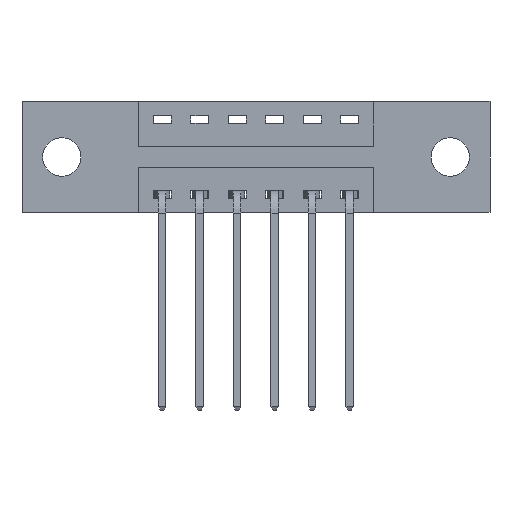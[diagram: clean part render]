
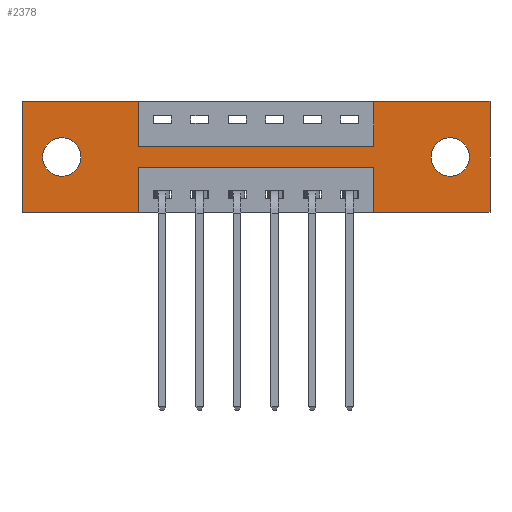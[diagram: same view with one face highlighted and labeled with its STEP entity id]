
A CAD part, front view. The second image highlights one B-rep face of the part: STEP entity #2378.
In plain terms, the highlighted planar face has unit normal (0, -1, 0).
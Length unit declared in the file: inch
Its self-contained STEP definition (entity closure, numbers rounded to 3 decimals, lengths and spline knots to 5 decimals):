
#19 = DIRECTION ( 'NONE',  ( 0., 0., -1. ) ) ;
#32 = CARTESIAN_POINT ( 'NONE',  ( 0., 0., -0.37 ) ) ;
#41 = VERTEX_POINT ( 'NONE', #8412 ) ;
#143 = CARTESIAN_POINT ( 'NONE',  ( 0.1325, 0., -0.249 ) ) ;
#238 = VERTEX_POINT ( 'NONE', #3917 ) ;
#343 = DIRECTION ( 'NONE',  ( 0., 1., 0. ) ) ;
#346 = VERTEX_POINT ( 'NONE', #7592 ) ;
#360 = ORIENTED_EDGE ( 'NONE', *, *, #2982, .F. ) ;
#462 = VERTEX_POINT ( 'NONE', #5036 ) ;
#473 = VERTEX_POINT ( 'NONE', #32 ) ;
#521 = CARTESIAN_POINT ( 'NONE',  ( 0.3875, 0., -0.37 ) ) ;
#602 = VERTEX_POINT ( 'NONE', #2443 ) ;
#650 = ORIENTED_EDGE ( 'NONE', *, *, #7500, .F. ) ;
#718 = LINE ( 'NONE', #4218, #4703 ) ;
#729 = CARTESIAN_POINT ( 'NONE',  ( 1.1725, 0., 0. ) ) ;
#827 = PLANE ( 'NONE',  #6484 ) ;
#828 = LINE ( 'NONE', #2027, #6202 ) ;
#871 = CARTESIAN_POINT ( 'NONE',  ( 0.1325, 0., -0.185 ) ) ;
#906 = DIRECTION ( 'NONE',  ( 0., 0., 1. ) ) ;
#968 = EDGE_LOOP ( 'NONE', ( #5894, #3913 ) ) ;
#1133 = CIRCLE ( 'NONE', #2251, 0.064 ) ;
#1312 = CARTESIAN_POINT ( 'NONE',  ( 1.4275, 0., -0.185 ) ) ;
#1410 = DIRECTION ( 'NONE',  ( 0., 0., -1. ) ) ;
#1457 = DIRECTION ( 'NONE',  ( -1., 0., 0. ) ) ;
#1524 = VERTEX_POINT ( 'NONE', #3330 ) ;
#1532 = EDGE_CURVE ( 'NONE', #238, #2907, #2862, .T. ) ;
#1658 = EDGE_CURVE ( 'NONE', #346, #1524, #1133, .T. ) ;
#1660 = DIRECTION ( 'NONE',  ( -1., 0., 0. ) ) ;
#1737 = CARTESIAN_POINT ( 'NONE',  ( 0., 0., -0.37 ) ) ;
#1757 = EDGE_CURVE ( 'NONE', #41, #2818, #7051, .T. ) ;
#1808 = DIRECTION ( 'NONE',  ( 0., 1., 0. ) ) ;
#1864 = ORIENTED_EDGE ( 'NONE', *, *, #4848, .F. ) ;
#1951 = LINE ( 'NONE', #7904, #2161 ) ;
#1965 = CIRCLE ( 'NONE', #3272, 0.064 ) ;
#1988 = LINE ( 'NONE', #7984, #6929 ) ;
#2027 = CARTESIAN_POINT ( 'NONE',  ( 0., 0., -0.37 ) ) ;
#2107 = CARTESIAN_POINT ( 'NONE',  ( 0., 0., -0.37 ) ) ;
#2161 = VECTOR ( 'NONE', #5864, 39.37008 ) ;
#2176 = VECTOR ( 'NONE', #5991, 39.37008 ) ;
#2251 = AXIS2_PLACEMENT_3D ( 'NONE', #5370, #4902, #1410 ) ;
#2328 = LINE ( 'NONE', #3090, #6091 ) ;
#2378 = ADVANCED_FACE ( 'NONE', ( #5490, #8020, #8178 ), #827, .T. ) ;
#2443 = CARTESIAN_POINT ( 'NONE',  ( 1.56, 0., 0. ) ) ;
#2446 = ORIENTED_EDGE ( 'NONE', *, *, #7838, .F. ) ;
#2808 = CARTESIAN_POINT ( 'NONE',  ( 0.3875, 0., -0.37 ) ) ;
#2818 = VERTEX_POINT ( 'NONE', #143 ) ;
#2862 = LINE ( 'NONE', #2808, #4669 ) ;
#2907 = VERTEX_POINT ( 'NONE', #521 ) ;
#2909 = VERTEX_POINT ( 'NONE', #5885 ) ;
#2913 = EDGE_CURVE ( 'NONE', #2818, #41, #1965, .T. ) ;
#2922 = LINE ( 'NONE', #6301, #4426 ) ;
#2941 = CARTESIAN_POINT ( 'NONE',  ( 1.1725, 0., -0.15 ) ) ;
#2982 = EDGE_CURVE ( 'NONE', #2907, #473, #828, .T. ) ;
#3090 = CARTESIAN_POINT ( 'NONE',  ( 0.3875, 0., -0.22 ) ) ;
#3196 = VECTOR ( 'NONE', #3379, 39.37008 ) ;
#3270 = AXIS2_PLACEMENT_3D ( 'NONE', #871, #343, #7706 ) ;
#3272 = AXIS2_PLACEMENT_3D ( 'NONE', #7983, #5324, #4589 ) ;
#3289 = ORIENTED_EDGE ( 'NONE', *, *, #1757, .T. ) ;
#3330 = CARTESIAN_POINT ( 'NONE',  ( 1.4275, 0., -0.121 ) ) ;
#3357 = VERTEX_POINT ( 'NONE', #4298 ) ;
#3379 = DIRECTION ( 'NONE',  ( 0., 0., 1. ) ) ;
#3510 = LINE ( 'NONE', #729, #7216 ) ;
#3542 = EDGE_CURVE ( 'NONE', #3357, #602, #1988, .T. ) ;
#3668 = VERTEX_POINT ( 'NONE', #5072 ) ;
#3913 = ORIENTED_EDGE ( 'NONE', *, *, #1658, .T. ) ;
#3917 = CARTESIAN_POINT ( 'NONE',  ( 0.3875, 0., -0.22 ) ) ;
#3933 = LINE ( 'NONE', #5207, #2176 ) ;
#4116 = ORIENTED_EDGE ( 'NONE', *, *, #8415, .F. ) ;
#4216 = CARTESIAN_POINT ( 'NONE',  ( 1.1725, 0., -0.37 ) ) ;
#4218 = CARTESIAN_POINT ( 'NONE',  ( 0.3875, 0., 0. ) ) ;
#4272 = ORIENTED_EDGE ( 'NONE', *, *, #6572, .F. ) ;
#4298 = CARTESIAN_POINT ( 'NONE',  ( 1.1725, 0., 0. ) ) ;
#4302 = ORIENTED_EDGE ( 'NONE', *, *, #4427, .F. ) ;
#4332 = ORIENTED_EDGE ( 'NONE', *, *, #4473, .F. ) ;
#4426 = VECTOR ( 'NONE', #6876, 39.37008 ) ;
#4427 = EDGE_CURVE ( 'NONE', #2909, #5092, #718, .T. ) ;
#4473 = EDGE_CURVE ( 'NONE', #5092, #4674, #1951, .T. ) ;
#4528 = DIRECTION ( 'NONE',  ( 0., 0., -1. ) ) ;
#4554 = CARTESIAN_POINT ( 'NONE',  ( 0.3875, 0., -0.15 ) ) ;
#4589 = DIRECTION ( 'NONE',  ( 0., 0., 1. ) ) ;
#4669 = VECTOR ( 'NONE', #7443, 39.37008 ) ;
#4674 = VERTEX_POINT ( 'NONE', #2941 ) ;
#4703 = VECTOR ( 'NONE', #19, 39.37008 ) ;
#4848 = EDGE_CURVE ( 'NONE', #4674, #3357, #3510, .T. ) ;
#4859 = DIRECTION ( 'NONE',  ( 1., 0., 0. ) ) ;
#4902 = DIRECTION ( 'NONE',  ( 0., 1., 0. ) ) ;
#4943 = EDGE_CURVE ( 'NONE', #1524, #346, #8605, .T. ) ;
#5036 = CARTESIAN_POINT ( 'NONE',  ( 1.1725, 0., -0.22 ) ) ;
#5072 = CARTESIAN_POINT ( 'NONE',  ( 1.56, 0., -0.37 ) ) ;
#5092 = VERTEX_POINT ( 'NONE', #4554 ) ;
#5181 = VERTEX_POINT ( 'NONE', #7384 ) ;
#5207 = CARTESIAN_POINT ( 'NONE',  ( 1.56, 0., 0. ) ) ;
#5274 = LINE ( 'NONE', #5970, #3196 ) ;
#5310 = EDGE_LOOP ( 'NONE', ( #6401, #650, #2446, #8100, #4116, #6110, #1864, #4332, #4302, #4272, #8432, #360 ) ) ;
#5324 = DIRECTION ( 'NONE',  ( 0., 1., 0. ) ) ;
#5344 = VERTEX_POINT ( 'NONE', #6457 ) ;
#5370 = CARTESIAN_POINT ( 'NONE',  ( 1.4275, 0., -0.185 ) ) ;
#5454 = DIRECTION ( 'NONE',  ( 0., -1., 0. ) ) ;
#5473 = DIRECTION ( 'NONE',  ( 0., 0., 1. ) ) ;
#5490 = FACE_BOUND ( 'NONE', #968, .T. ) ;
#5609 = LINE ( 'NONE', #4216, #6805 ) ;
#5845 = LINE ( 'NONE', #1737, #8636 ) ;
#5864 = DIRECTION ( 'NONE',  ( 1., 0., 0. ) ) ;
#5885 = CARTESIAN_POINT ( 'NONE',  ( 0.3875, 0., 0. ) ) ;
#5894 = ORIENTED_EDGE ( 'NONE', *, *, #4943, .T. ) ;
#5970 = CARTESIAN_POINT ( 'NONE',  ( 0., 0., 0. ) ) ;
#5991 = DIRECTION ( 'NONE',  ( 0., 0., -1. ) ) ;
#6091 = VECTOR ( 'NONE', #1660, 39.37008 ) ;
#6110 = ORIENTED_EDGE ( 'NONE', *, *, #3542, .F. ) ;
#6202 = VECTOR ( 'NONE', #1457, 39.37008 ) ;
#6301 = CARTESIAN_POINT ( 'NONE',  ( 0., 0., 0. ) ) ;
#6401 = ORIENTED_EDGE ( 'NONE', *, *, #1532, .F. ) ;
#6457 = CARTESIAN_POINT ( 'NONE',  ( 1.1725, 0., -0.37 ) ) ;
#6484 = AXIS2_PLACEMENT_3D ( 'NONE', #2107, #5454, #8126 ) ;
#6572 = EDGE_CURVE ( 'NONE', #5181, #2909, #2922, .T. ) ;
#6703 = ORIENTED_EDGE ( 'NONE', *, *, #2913, .T. ) ;
#6805 = VECTOR ( 'NONE', #5473, 39.37008 ) ;
#6876 = DIRECTION ( 'NONE',  ( 1., 0., 0. ) ) ;
#6929 = VECTOR ( 'NONE', #4859, 39.37008 ) ;
#7051 = CIRCLE ( 'NONE', #3270, 0.064 ) ;
#7094 = AXIS2_PLACEMENT_3D ( 'NONE', #1312, #1808, #4528 ) ;
#7216 = VECTOR ( 'NONE', #906, 39.37008 ) ;
#7384 = CARTESIAN_POINT ( 'NONE',  ( 0., 0., 0. ) ) ;
#7443 = DIRECTION ( 'NONE',  ( 0., 0., -1. ) ) ;
#7500 = EDGE_CURVE ( 'NONE', #462, #238, #2328, .T. ) ;
#7592 = CARTESIAN_POINT ( 'NONE',  ( 1.4275, 0., -0.249 ) ) ;
#7706 = DIRECTION ( 'NONE',  ( 0., 0., 1. ) ) ;
#7838 = EDGE_CURVE ( 'NONE', #5344, #462, #5609, .T. ) ;
#7904 = CARTESIAN_POINT ( 'NONE',  ( 0.3875, 0., -0.15 ) ) ;
#7983 = CARTESIAN_POINT ( 'NONE',  ( 0.1325, 0., -0.185 ) ) ;
#7984 = CARTESIAN_POINT ( 'NONE',  ( 0., 0., 0. ) ) ;
#8020 = FACE_BOUND ( 'NONE', #8242, .T. ) ;
#8100 = ORIENTED_EDGE ( 'NONE', *, *, #8589, .F. ) ;
#8126 = DIRECTION ( 'NONE',  ( 0., 0., -1. ) ) ;
#8178 = FACE_OUTER_BOUND ( 'NONE', #5310, .T. ) ;
#8242 = EDGE_LOOP ( 'NONE', ( #3289, #6703 ) ) ;
#8412 = CARTESIAN_POINT ( 'NONE',  ( 0.1325, 0., -0.121 ) ) ;
#8415 = EDGE_CURVE ( 'NONE', #602, #3668, #3933, .T. ) ;
#8432 = ORIENTED_EDGE ( 'NONE', *, *, #8675, .F. ) ;
#8443 = DIRECTION ( 'NONE',  ( -1., 0., 0. ) ) ;
#8589 = EDGE_CURVE ( 'NONE', #3668, #5344, #5845, .T. ) ;
#8605 = CIRCLE ( 'NONE', #7094, 0.064 ) ;
#8636 = VECTOR ( 'NONE', #8443, 39.37008 ) ;
#8675 = EDGE_CURVE ( 'NONE', #473, #5181, #5274, .T. ) ;
